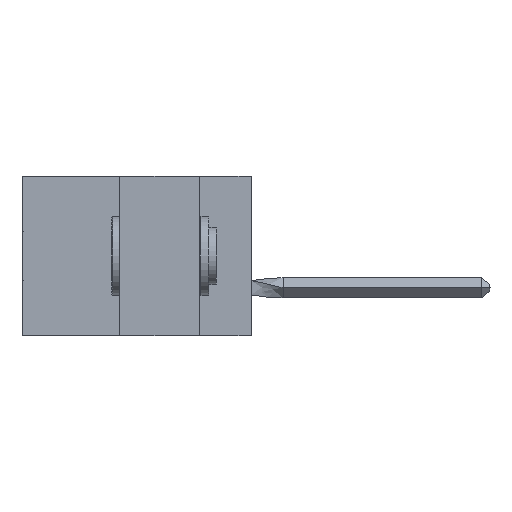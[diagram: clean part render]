
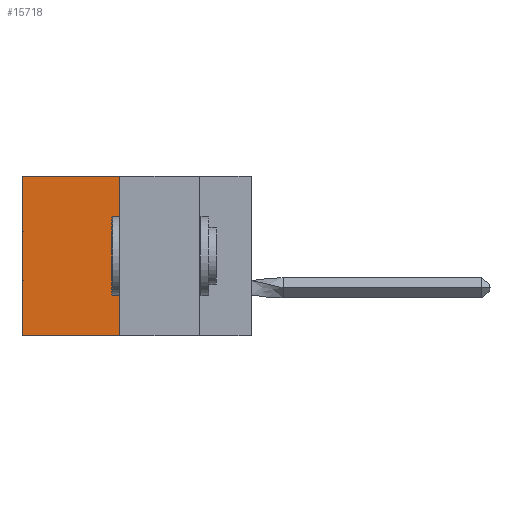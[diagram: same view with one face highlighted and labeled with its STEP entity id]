
A CAD part, left-side view. The second image highlights one B-rep face of the part: STEP entity #15718.
In plain terms, the highlighted planar face has unit normal (-1, 0, 0).
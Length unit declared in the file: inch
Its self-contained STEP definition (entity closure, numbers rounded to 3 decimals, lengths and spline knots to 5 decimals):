
#737 = VERTEX_POINT ( 'NONE', #28759 ) ;
#3542 = CARTESIAN_POINT ( 'NONE',  ( 0.305, 0.413, -0.5 ) ) ;
#3642 = AXIS2_PLACEMENT_3D ( 'NONE', #42247, #13081, #8759 ) ;
#3716 = VERTEX_POINT ( 'NONE', #37242 ) ;
#3809 = VERTEX_POINT ( 'NONE', #15931 ) ;
#3812 = LINE ( 'NONE', #3542, #6653 ) ;
#5588 = CARTESIAN_POINT ( 'NONE',  ( 0.305, 0.72, -0.5 ) ) ;
#6653 = VECTOR ( 'NONE', #29203, 39.37008 ) ;
#8759 = DIRECTION ( 'NONE',  ( 0., 0., -1. ) ) ;
#13081 = DIRECTION ( 'NONE',  ( 1., 0., 0. ) ) ;
#13298 = DIRECTION ( 'NONE',  ( 0., 0., -1. ) ) ;
#14161 = VECTOR ( 'NONE', #41147, 39.37008 ) ;
#15718 = ADVANCED_FACE ( 'NONE', ( #29884 ), #20324, .F. ) ;
#15931 = CARTESIAN_POINT ( 'NONE',  ( 0.305, 0.413, -0.5 ) ) ;
#17637 = LINE ( 'NONE', #44816, #14161 ) ;
#18291 = VECTOR ( 'NONE', #44229, 39.37008 ) ;
#18681 = LINE ( 'NONE', #5588, #43269 ) ;
#18978 = EDGE_CURVE ( 'NONE', #3809, #737, #3812, .T. ) ;
#20324 = PLANE ( 'NONE',  #3642 ) ;
#26881 = CARTESIAN_POINT ( 'NONE',  ( 0.305, 0.72, 0. ) ) ;
#28759 = CARTESIAN_POINT ( 'NONE',  ( 0.305, 0.72, -0.5 ) ) ;
#28931 = VERTEX_POINT ( 'NONE', #26881 ) ;
#29203 = DIRECTION ( 'NONE',  ( 0., 1., 0. ) ) ;
#29884 = FACE_OUTER_BOUND ( 'NONE', #33052, .T. ) ;
#33052 = EDGE_LOOP ( 'NONE', ( #47430, #35740, #47211, #42206 ) ) ;
#34263 = EDGE_CURVE ( 'NONE', #3716, #3809, #40042, .T. ) ;
#34916 = EDGE_CURVE ( 'NONE', #3716, #28931, #17637, .T. ) ;
#35740 = ORIENTED_EDGE ( 'NONE', *, *, #18978, .F. ) ;
#36909 = CARTESIAN_POINT ( 'NONE',  ( 0.305, 0.413, -0.5 ) ) ;
#37242 = CARTESIAN_POINT ( 'NONE',  ( 0.305, 0.413, 0. ) ) ;
#40042 = LINE ( 'NONE', #36909, #18291 ) ;
#41147 = DIRECTION ( 'NONE',  ( 0., 1., 0. ) ) ;
#42206 = ORIENTED_EDGE ( 'NONE', *, *, #34916, .T. ) ;
#42247 = CARTESIAN_POINT ( 'NONE',  ( 0.305, 0.413, -0.5 ) ) ;
#43269 = VECTOR ( 'NONE', #13298, 39.37008 ) ;
#43487 = EDGE_CURVE ( 'NONE', #28931, #737, #18681, .T. ) ;
#44229 = DIRECTION ( 'NONE',  ( 0., 0., -1. ) ) ;
#44816 = CARTESIAN_POINT ( 'NONE',  ( 0.305, 0.413, 0. ) ) ;
#47211 = ORIENTED_EDGE ( 'NONE', *, *, #34263, .F. ) ;
#47430 = ORIENTED_EDGE ( 'NONE', *, *, #43487, .T. ) ;
